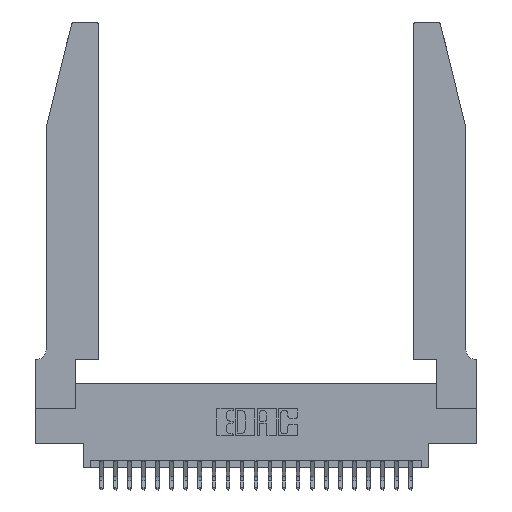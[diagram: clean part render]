
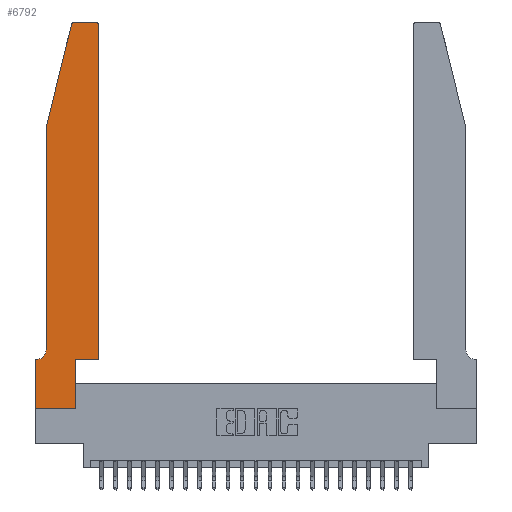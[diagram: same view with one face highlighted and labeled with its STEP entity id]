
A CAD part, top view. The second image highlights one B-rep face of the part: STEP entity #6792.
In plain terms, the highlighted planar face has unit normal (0, 0, 1).
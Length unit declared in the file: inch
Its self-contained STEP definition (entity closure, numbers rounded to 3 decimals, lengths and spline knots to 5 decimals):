
#141 = LINE ( 'NONE', #24408, #15638 ) ;
#218 = ORIENTED_EDGE ( 'NONE', *, *, #13079, .T. ) ;
#1127 = CARTESIAN_POINT ( 'NONE',  ( 0.25487, 2.72718, 0.37 ) ) ;
#1153 = VERTEX_POINT ( 'NONE', #9229 ) ;
#1166 = DIRECTION ( 'NONE',  ( 1., 0., 0. ) ) ;
#1217 = CARTESIAN_POINT ( 'NONE',  ( 0.2865, 0.35, 0.37 ) ) ;
#1318 = EDGE_CURVE ( 'NONE', #17051, #2175, #141, .T. ) ;
#1845 = CARTESIAN_POINT ( 'NONE',  ( 0., 0., 0.37 ) ) ;
#2175 = VERTEX_POINT ( 'NONE', #13672 ) ;
#2204 = LINE ( 'NONE', #14070, #12964 ) ;
#2285 = VECTOR ( 'NONE', #11261, 39.37008 ) ;
#2658 = VERTEX_POINT ( 'NONE', #7370 ) ;
#2946 = LINE ( 'NONE', #13080, #2285 ) ;
#3054 = CARTESIAN_POINT ( 'NONE',  ( 0., 0., 0.37 ) ) ;
#3145 = AXIS2_PLACEMENT_3D ( 'NONE', #6712, #22338, #10731 ) ;
#3211 = VERTEX_POINT ( 'NONE', #3054 ) ;
#3467 = EDGE_CURVE ( 'NONE', #15568, #3211, #10827, .T. ) ;
#3791 = VERTEX_POINT ( 'NONE', #18645 ) ;
#4229 = CIRCLE ( 'NONE', #9656, 0.07 ) ;
#4570 = VERTEX_POINT ( 'NONE', #15016 ) ;
#4620 = ORIENTED_EDGE ( 'NONE', *, *, #1318, .T. ) ;
#4671 = PLANE ( 'NONE',  #3145 ) ;
#4992 = DIRECTION ( 'NONE',  ( 0., 0., 1. ) ) ;
#5433 = ORIENTED_EDGE ( 'NONE', *, *, #23719, .T. ) ;
#5530 = EDGE_CURVE ( 'NONE', #7955, #8412, #8188, .T. ) ;
#5537 = LINE ( 'NONE', #11963, #11651 ) ;
#6081 = EDGE_CURVE ( 'NONE', #2175, #6523, #21894, .T. ) ;
#6523 = VERTEX_POINT ( 'NONE', #9882 ) ;
#6712 = CARTESIAN_POINT ( 'NONE',  ( 0., 0.35, 0.37 ) ) ;
#6792 = ADVANCED_FACE ( 'NONE', ( #12509 ), #4671, .T. ) ;
#6905 = CARTESIAN_POINT ( 'NONE',  ( 0.4505, 0.35, 0.37 ) ) ;
#7370 = CARTESIAN_POINT ( 'NONE',  ( 0.2865, 0., 0.37 ) ) ;
#7673 = EDGE_LOOP ( 'NONE', ( #12548, #5433, #9441, #19030, #218, #9541, #25558, #7699, #24539, #25398, #4620, #19212 ) ) ;
#7699 = ORIENTED_EDGE ( 'NONE', *, *, #8562, .T. ) ;
#7734 = CARTESIAN_POINT ( 'NONE',  ( 0., 0.35, 0.37 ) ) ;
#7955 = VERTEX_POINT ( 'NONE', #1127 ) ;
#8188 = LINE ( 'NONE', #20774, #18030 ) ;
#8412 = VERTEX_POINT ( 'NONE', #14804 ) ;
#8562 = EDGE_CURVE ( 'NONE', #3211, #2658, #2946, .T. ) ;
#8602 = VECTOR ( 'NONE', #1166, 39.37008 ) ;
#8749 = CARTESIAN_POINT ( 'NONE',  ( 0.4205, 2.72, 0.37 ) ) ;
#9229 = CARTESIAN_POINT ( 'NONE',  ( 0.0055, 0.35, 0.37 ) ) ;
#9441 = ORIENTED_EDGE ( 'NONE', *, *, #5530, .T. ) ;
#9541 = ORIENTED_EDGE ( 'NONE', *, *, #22304, .T. ) ;
#9656 = AXIS2_PLACEMENT_3D ( 'NONE', #22890, #11289, #24856 ) ;
#9780 = VERTEX_POINT ( 'NONE', #20582 ) ;
#9882 = CARTESIAN_POINT ( 'NONE',  ( 0.4205, 2.75, 0.37 ) ) ;
#10731 = DIRECTION ( 'NONE',  ( 1., 0., 0. ) ) ;
#10760 = DIRECTION ( 'NONE',  ( 1., 0., 0. ) ) ;
#10827 = LINE ( 'NONE', #1845, #15439 ) ;
#11261 = DIRECTION ( 'NONE',  ( 1., 0., 0. ) ) ;
#11289 = DIRECTION ( 'NONE',  ( 0., 0., -1. ) ) ;
#11651 = VECTOR ( 'NONE', #13960, 39.37008 ) ;
#11963 = CARTESIAN_POINT ( 'NONE',  ( 0.0755, 0.35, 0.37 ) ) ;
#12509 = FACE_OUTER_BOUND ( 'NONE', #7673, .T. ) ;
#12548 = ORIENTED_EDGE ( 'NONE', *, *, #16156, .T. ) ;
#12964 = VECTOR ( 'NONE', #25631, 39.37008 ) ;
#13079 = EDGE_CURVE ( 'NONE', #3791, #1153, #4229, .T. ) ;
#13080 = CARTESIAN_POINT ( 'NONE',  ( 0., 0., 0.37 ) ) ;
#13291 = LINE ( 'NONE', #13310, #8602 ) ;
#13310 = CARTESIAN_POINT ( 'NONE',  ( 0.4505, 0.35, 0.37 ) ) ;
#13672 = CARTESIAN_POINT ( 'NONE',  ( 0.4505, 2.72, 0.37 ) ) ;
#13960 = DIRECTION ( 'NONE',  ( -1., 0., 0. ) ) ;
#14070 = CARTESIAN_POINT ( 'NONE',  ( 0.0755, 2., 0.37 ) ) ;
#14804 = CARTESIAN_POINT ( 'NONE',  ( 0.0755, 2., 0.37 ) ) ;
#15016 = CARTESIAN_POINT ( 'NONE',  ( 0.284, 2.75, 0.37 ) ) ;
#15113 = AXIS2_PLACEMENT_3D ( 'NONE', #16856, #4992, #18779 ) ;
#15430 = CIRCLE ( 'NONE', #15113, 0.03 ) ;
#15439 = VECTOR ( 'NONE', #17827, 39.37008 ) ;
#15568 = VERTEX_POINT ( 'NONE', #7734 ) ;
#15638 = VECTOR ( 'NONE', #24264, 39.37008 ) ;
#16014 = DIRECTION ( 'NONE',  ( -1., 0., 0. ) ) ;
#16156 = EDGE_CURVE ( 'NONE', #6523, #4570, #23158, .T. ) ;
#16856 = CARTESIAN_POINT ( 'NONE',  ( 0.284, 2.72, 0.37 ) ) ;
#17051 = VERTEX_POINT ( 'NONE', #6905 ) ;
#17827 = DIRECTION ( 'NONE',  ( 0., -1., 0. ) ) ;
#18030 = VECTOR ( 'NONE', #22740, 39.37008 ) ;
#18645 = CARTESIAN_POINT ( 'NONE',  ( 0.0755, 0.42, 0.37 ) ) ;
#18779 = DIRECTION ( 'NONE',  ( 1., 0., 0. ) ) ;
#19030 = ORIENTED_EDGE ( 'NONE', *, *, #20927, .T. ) ;
#19212 = ORIENTED_EDGE ( 'NONE', *, *, #6081, .T. ) ;
#20454 = VECTOR ( 'NONE', #24923, 39.37008 ) ;
#20582 = CARTESIAN_POINT ( 'NONE',  ( 0.2865, 0.35, 0.37 ) ) ;
#20653 = EDGE_CURVE ( 'NONE', #9780, #17051, #13291, .T. ) ;
#20774 = CARTESIAN_POINT ( 'NONE',  ( 0.0755, 2., 0.37 ) ) ;
#20927 = EDGE_CURVE ( 'NONE', #8412, #3791, #2204, .T. ) ;
#21056 = LINE ( 'NONE', #1217, #20454 ) ;
#21894 = CIRCLE ( 'NONE', #25407, 0.03 ) ;
#22304 = EDGE_CURVE ( 'NONE', #1153, #15568, #5537, .T. ) ;
#22338 = DIRECTION ( 'NONE',  ( 0., 0., 1. ) ) ;
#22369 = DIRECTION ( 'NONE',  ( 0., 0., 1. ) ) ;
#22555 = VECTOR ( 'NONE', #16014, 39.37008 ) ;
#22740 = DIRECTION ( 'NONE',  ( -0.239, -0.971, 0. ) ) ;
#22890 = CARTESIAN_POINT ( 'NONE',  ( 0.0055, 0.42, 0.37 ) ) ;
#23158 = LINE ( 'NONE', #25639, #22555 ) ;
#23719 = EDGE_CURVE ( 'NONE', #4570, #7955, #15430, .T. ) ;
#24264 = DIRECTION ( 'NONE',  ( 0., 1., 0. ) ) ;
#24408 = CARTESIAN_POINT ( 'NONE',  ( 0.4505, 0.35, 0.37 ) ) ;
#24539 = ORIENTED_EDGE ( 'NONE', *, *, #25384, .T. ) ;
#24856 = DIRECTION ( 'NONE',  ( -1., 0., 0. ) ) ;
#24923 = DIRECTION ( 'NONE',  ( 0., 1., 0. ) ) ;
#25384 = EDGE_CURVE ( 'NONE', #2658, #9780, #21056, .T. ) ;
#25398 = ORIENTED_EDGE ( 'NONE', *, *, #20653, .T. ) ;
#25407 = AXIS2_PLACEMENT_3D ( 'NONE', #8749, #22369, #10760 ) ;
#25558 = ORIENTED_EDGE ( 'NONE', *, *, #3467, .T. ) ;
#25631 = DIRECTION ( 'NONE',  ( 0., -1., 0. ) ) ;
#25639 = CARTESIAN_POINT ( 'NONE',  ( 0.2605, 2.75, 0.37 ) ) ;
